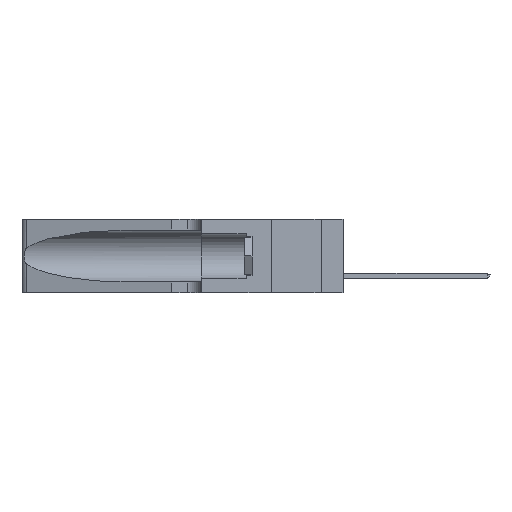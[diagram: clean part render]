
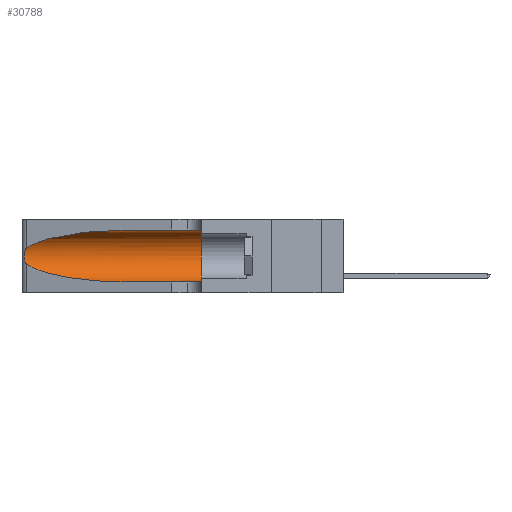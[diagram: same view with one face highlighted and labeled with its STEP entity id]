
A CAD part, left-side view. The second image highlights one B-rep face of the part: STEP entity #30788.
In plain terms, the highlighted cylindrical face has radius 3.308 mm (diameter 6.617 mm), a partial arc.
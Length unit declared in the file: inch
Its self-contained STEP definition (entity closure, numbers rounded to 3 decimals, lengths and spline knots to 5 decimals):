
#415 = CIRCLE ( 'NONE', #22055, 0.13025 ) ;
#2129 = CARTESIAN_POINT ( 'NONE',  ( 0.25789, 1.23486, 0.15765 ) ) ;
#2946 = CARTESIAN_POINT ( 'NONE',  ( 0.1305, 0.35, 0.05475 ) ) ;
#3650 = CARTESIAN_POINT ( 'NONE',  ( 0.18966, 0.96281, 0.05475 ) ) ;
#5590 = CARTESIAN_POINT ( 'NONE',  ( 0.25487, 1.22718, 0.22369 ) ) ;
#6288 = EDGE_CURVE ( 'NONE', #25862, #20808, #42321, .T. ) ;
#6908 = CARTESIAN_POINT ( 'NONE',  ( 0.1305, 0.72297, 0.31525 ) ) ;
#8221 = ORIENTED_EDGE ( 'NONE', *, *, #46104, .F. ) ;
#11296 = EDGE_CURVE ( 'NONE', #43976, #25862, #26006, .T. ) ;
#11717 = FACE_OUTER_BOUND ( 'NONE', #13345, .T. ) ;
#12519 = CARTESIAN_POINT ( 'NONE',  ( 0.25555, 1.22994, 0.2215 ) ) ;
#12967 = CARTESIAN_POINT ( 'NONE',  ( 0.1305, 0.35, 0.185 ) ) ;
#13345 = EDGE_LOOP ( 'NONE', ( #23470, #38823, #14655, #33266, #39003, #8221 ) ) ;
#14655 = ORIENTED_EDGE ( 'NONE', *, *, #6288, .T. ) ;
#14894 = DIRECTION ( 'NONE',  ( 0., -1., 0. ) ) ;
#15629 = CARTESIAN_POINT ( 'NONE',  ( 0.25487, 1.22718, 0.22369 ) ) ;
#15967 = CARTESIAN_POINT ( 'NONE',  ( 0.25854, 1.2359, 0.20912 ) ) ;
#16653 = VERTEX_POINT ( 'NONE', #2946 ) ;
#17685 = CARTESIAN_POINT ( 'NONE',  ( 0.25487, 1.22718, 0.14631 ) ) ;
#18972 = CARTESIAN_POINT ( 'NONE',  ( 0.1305, 1.61858, 0.185 ) ) ;
#19903 = CARTESIAN_POINT ( 'NONE',  ( 0.26018, 1.23835, 0.19895 ) ) ;
#20078 = CARTESIAN_POINT ( 'NONE',  ( 0.26017, 1.23833, 0.17102 ) ) ;
#20329 = VECTOR ( 'NONE', #28630, 39.37008 ) ;
#20808 = VERTEX_POINT ( 'NONE', #40694 ) ;
#20894 = VERTEX_POINT ( 'NONE', #45772 ) ;
#21470 = CARTESIAN_POINT ( 'NONE',  ( 0.1305, 0.72297, 0.05475 ) ) ;
#22055 = AXIS2_PLACEMENT_3D ( 'NONE', #12967, #43899, #30128 ) ;
#23354 = CARTESIAN_POINT ( 'NONE',  ( 0.25487, 1.22718, 0.14631 ) ) ;
#23470 = ORIENTED_EDGE ( 'NONE', *, *, #34953, .T. ) ;
#23653 = EDGE_CURVE ( 'NONE', #20894, #16653, #415, .T. ) ;
#23697 = CARTESIAN_POINT ( 'NONE',  ( 0.25856, 1.23593, 0.16098 ) ) ;
#25458 = CARTESIAN_POINT ( 'NONE',  ( 0.1305, 0.72297, 0.31525 ) ) ;
#25862 = VERTEX_POINT ( 'NONE', #23354 ) ;
#26006 = B_SPLINE_CURVE_WITH_KNOTS ( 'NONE', 3,
 ( #41442, #12519, #41599, #34330, #15967, #19903, #27192, #30834, #20078, #23697, #2129, #27351, #31010, #34666 ),
 .UNSPECIFIED., .F., .F.,
 ( 4, 2, 2, 2, 2, 2, 4 ),
 ( 0., 0.00027, 0.00053, 0.00107, 0.0016, 0.00187, 0.00214 ),
 .UNSPECIFIED. ) ;
#27192 = CARTESIAN_POINT ( 'NONE',  ( 0.26075, 1.23896, 0.19203 ) ) ;
#27351 = CARTESIAN_POINT ( 'NONE',  ( 0.25639, 1.23186, 0.15144 ) ) ;
#28630 = DIRECTION ( 'NONE',  ( 0., -1., 0. ) ) ;
#28720 = CYLINDRICAL_SURFACE ( 'NONE', #45566, 0.13025 ) ;
#30128 = DIRECTION ( 'NONE',  ( 0., 0., 1. ) ) ;
#30788 = ADVANCED_FACE ( 'NONE', ( #11717 ), #28720, .F. ) ;
#30834 = CARTESIAN_POINT ( 'NONE',  ( 0.26075, 1.23896, 0.178 ) ) ;
#31010 = CARTESIAN_POINT ( 'NONE',  ( 0.25555, 1.22993, 0.14849 ) ) ;
#31501 = CARTESIAN_POINT ( 'NONE',  ( 0.2373, 1.15595, 0.28018 ) ) ;
#32288 = CARTESIAN_POINT ( 'NONE',  ( 0.1305, 1.61858, 0.05475 ) ) ;
#33266 = ORIENTED_EDGE ( 'NONE', *, *, #39783, .T. ) ;
#34330 = CARTESIAN_POINT ( 'NONE',  ( 0.25787, 1.23484, 0.2124 ) ) ;
#34666 = CARTESIAN_POINT ( 'NONE',  ( 0.25487, 1.22718, 0.14631 ) ) ;
#34953 = EDGE_CURVE ( 'NONE', #37601, #43976, #36490, .T. ) ;
#36490 =( BOUNDED_CURVE ( )  B_SPLINE_CURVE ( 3, ( #25458, #46496, #31501, #15629 ),
 .UNSPECIFIED., .F., .T. ) 
 B_SPLINE_CURVE_WITH_KNOTS ( ( 4, 4 ),
 ( 1.5708, 2.84003 ),
 .UNSPECIFIED. ) 
 CURVE ( )  GEOMETRIC_REPRESENTATION_ITEM ( )  RATIONAL_B_SPLINE_CURVE ( ( 1., 0.87, 0.87, 1. ) ) 
 REPRESENTATION_ITEM ( '' )  );
#37601 = VERTEX_POINT ( 'NONE', #6908 ) ;
#37623 = CARTESIAN_POINT ( 'NONE',  ( 0.1305, 1.61858, 0.31525 ) ) ;
#38823 = ORIENTED_EDGE ( 'NONE', *, *, #11296, .T. ) ;
#39003 = ORIENTED_EDGE ( 'NONE', *, *, #23653, .F. ) ;
#39685 = CARTESIAN_POINT ( 'NONE',  ( 0.2373, 1.15595, 0.08982 ) ) ;
#39783 = EDGE_CURVE ( 'NONE', #20808, #16653, #42999, .T. ) ;
#40216 = DIRECTION ( 'NONE',  ( 0., 0., -1. ) ) ;
#40587 = VECTOR ( 'NONE', #45160, 39.37008 ) ;
#40694 = CARTESIAN_POINT ( 'NONE',  ( 0.1305, 0.72297, 0.05475 ) ) ;
#41442 = CARTESIAN_POINT ( 'NONE',  ( 0.25487, 1.22718, 0.22369 ) ) ;
#41599 = CARTESIAN_POINT ( 'NONE',  ( 0.25639, 1.23184, 0.21858 ) ) ;
#42321 =( BOUNDED_CURVE ( )  B_SPLINE_CURVE ( 3, ( #17685, #39685, #3650, #21470 ),
 .UNSPECIFIED., .F., .F. ) 
 B_SPLINE_CURVE_WITH_KNOTS ( ( 4, 4 ),
 ( 3.44316, 4.71239 ),
 .UNSPECIFIED. ) 
 CURVE ( )  GEOMETRIC_REPRESENTATION_ITEM ( )  RATIONAL_B_SPLINE_CURVE ( ( 1., 0.87, 0.87, 1. ) ) 
 REPRESENTATION_ITEM ( '' )  );
#42890 = LINE ( 'NONE', #37623, #40587 ) ;
#42999 = LINE ( 'NONE', #32288, #20329 ) ;
#43899 = DIRECTION ( 'NONE',  ( 0., 1., 0. ) ) ;
#43976 = VERTEX_POINT ( 'NONE', #5590 ) ;
#45160 = DIRECTION ( 'NONE',  ( 0., -1., 0. ) ) ;
#45566 = AXIS2_PLACEMENT_3D ( 'NONE', #18972, #14894, #40216 ) ;
#45772 = CARTESIAN_POINT ( 'NONE',  ( 0.1305, 0.35, 0.31525 ) ) ;
#46104 = EDGE_CURVE ( 'NONE', #37601, #20894, #42890, .T. ) ;
#46496 = CARTESIAN_POINT ( 'NONE',  ( 0.18966, 0.96281, 0.31525 ) ) ;
